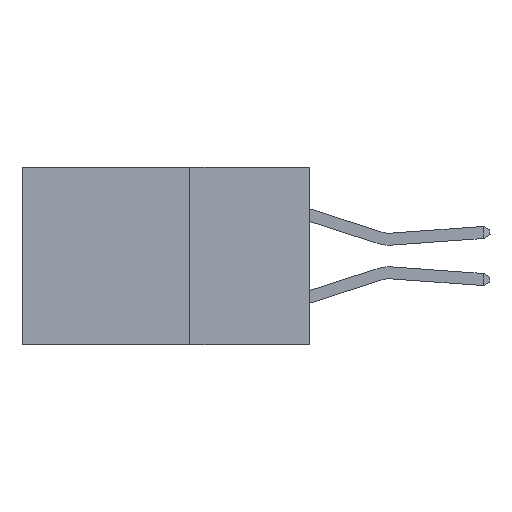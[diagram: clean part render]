
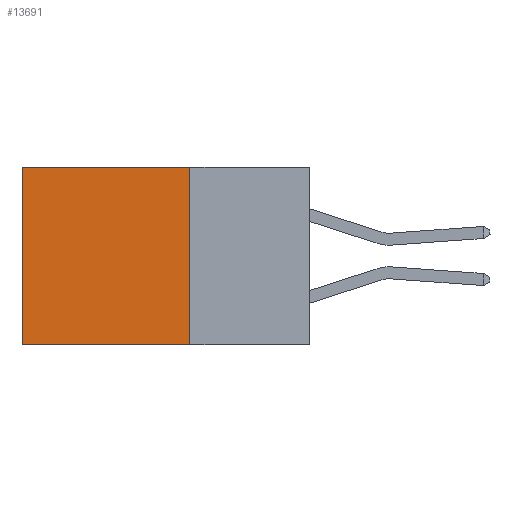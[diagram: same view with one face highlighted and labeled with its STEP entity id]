
A CAD part, left-side view. The second image highlights one B-rep face of the part: STEP entity #13691.
In plain terms, the highlighted planar face has unit normal (-1, 0, 0).
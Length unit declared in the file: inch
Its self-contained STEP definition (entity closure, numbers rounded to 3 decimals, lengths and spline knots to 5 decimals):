
#270 = EDGE_CURVE ( 'NONE', #3472, #11385, #14831, .T. ) ;
#1437 = VERTEX_POINT ( 'NONE', #12679 ) ;
#1556 = EDGE_CURVE ( 'NONE', #1437, #9922, #4772, .T. ) ;
#2322 = CARTESIAN_POINT ( 'NONE',  ( 0.2615, 0.25, 0. ) ) ;
#2328 = PLANE ( 'NONE',  #13052 ) ;
#2366 = CARTESIAN_POINT ( 'NONE',  ( 0.2615, 0.25, -0.37 ) ) ;
#2654 = CARTESIAN_POINT ( 'NONE',  ( 0.2615, 0.25, 0. ) ) ;
#2853 = CARTESIAN_POINT ( 'NONE',  ( 0.2615, 0.25, -0.37 ) ) ;
#3472 = VERTEX_POINT ( 'NONE', #2654 ) ;
#3538 = DIRECTION ( 'NONE',  ( 1., 0., 0. ) ) ;
#4208 = CARTESIAN_POINT ( 'NONE',  ( 0.2615, 0.6, -0.37 ) ) ;
#4560 = DIRECTION ( 'NONE',  ( 0., 0., -1. ) ) ;
#4772 = LINE ( 'NONE', #2366, #5122 ) ;
#5005 = EDGE_CURVE ( 'NONE', #3472, #1437, #12220, .T. ) ;
#5122 = VECTOR ( 'NONE', #12306, 39.37008 ) ;
#6080 = VECTOR ( 'NONE', #14948, 39.37008 ) ;
#7159 = DIRECTION ( 'NONE',  ( 0., 0., -1. ) ) ;
#7259 = CARTESIAN_POINT ( 'NONE',  ( 0.2615, 0.6, -0.37 ) ) ;
#7475 = ORIENTED_EDGE ( 'NONE', *, *, #9421, .T. ) ;
#9211 = LINE ( 'NONE', #7259, #11878 ) ;
#9256 = FACE_OUTER_BOUND ( 'NONE', #11714, .T. ) ;
#9344 = ORIENTED_EDGE ( 'NONE', *, *, #270, .T. ) ;
#9421 = EDGE_CURVE ( 'NONE', #11385, #9922, #9211, .T. ) ;
#9921 = CARTESIAN_POINT ( 'NONE',  ( 0.2615, 0.6, 0. ) ) ;
#9922 = VERTEX_POINT ( 'NONE', #4208 ) ;
#10454 = CARTESIAN_POINT ( 'NONE',  ( 0.2615, 0.25, -0.37 ) ) ;
#10470 = ORIENTED_EDGE ( 'NONE', *, *, #5005, .F. ) ;
#11192 = ORIENTED_EDGE ( 'NONE', *, *, #1556, .F. ) ;
#11385 = VERTEX_POINT ( 'NONE', #9921 ) ;
#11609 = DIRECTION ( 'NONE',  ( 0., 0., -1. ) ) ;
#11714 = EDGE_LOOP ( 'NONE', ( #7475, #11192, #10470, #9344 ) ) ;
#11878 = VECTOR ( 'NONE', #7159, 39.37008 ) ;
#12220 = LINE ( 'NONE', #2853, #14866 ) ;
#12306 = DIRECTION ( 'NONE',  ( 0., 1., 0. ) ) ;
#12679 = CARTESIAN_POINT ( 'NONE',  ( 0.2615, 0.25, -0.37 ) ) ;
#13052 = AXIS2_PLACEMENT_3D ( 'NONE', #10454, #3538, #11609 ) ;
#13691 = ADVANCED_FACE ( 'NONE', ( #9256 ), #2328, .F. ) ;
#14831 = LINE ( 'NONE', #2322, #6080 ) ;
#14866 = VECTOR ( 'NONE', #4560, 39.37008 ) ;
#14948 = DIRECTION ( 'NONE',  ( 0., 1., 0. ) ) ;
